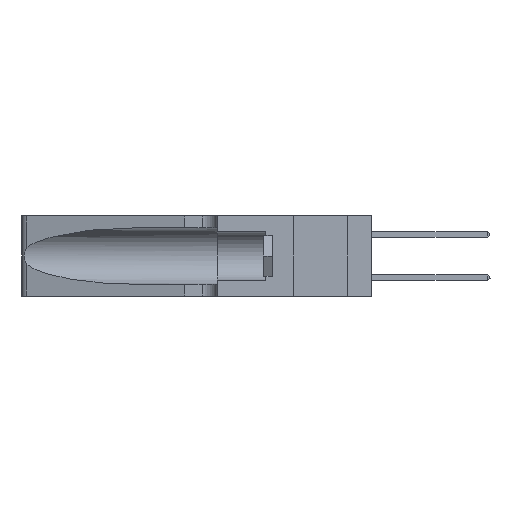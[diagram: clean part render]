
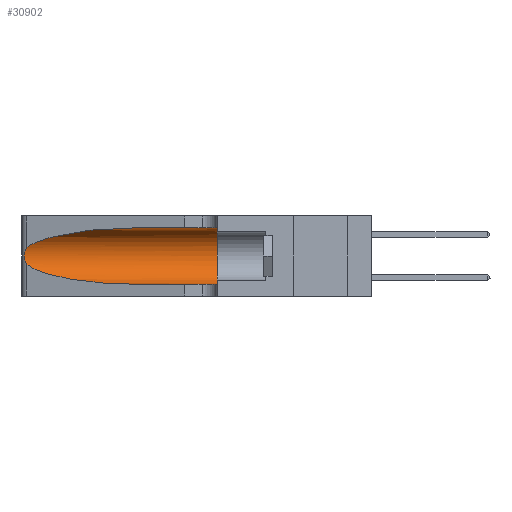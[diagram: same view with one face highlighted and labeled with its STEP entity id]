
A CAD part, left-side view. The second image highlights one B-rep face of the part: STEP entity #30902.
In plain terms, the highlighted cylindrical face has radius 3.308 mm (diameter 6.617 mm), a partial arc.
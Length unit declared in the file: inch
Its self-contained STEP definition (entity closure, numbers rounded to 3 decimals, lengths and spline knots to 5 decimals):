
#442 = AXIS2_PLACEMENT_3D ( 'NONE', #27284, #17613, #19500 ) ;
#1163 = VERTEX_POINT ( 'NONE', #16244 ) ;
#1257 = CARTESIAN_POINT ( 'NONE',  ( 0.25639, 1.23184, 0.21858 ) ) ;
#1404 = CARTESIAN_POINT ( 'NONE',  ( 0.18966, 0.96281, 0.31525 ) ) ;
#1647 = CARTESIAN_POINT ( 'NONE',  ( 0.1305, 0.35, 0.05475 ) ) ;
#2185 = DIRECTION ( 'NONE',  ( 0., -1., 0. ) ) ;
#2292 = ORIENTED_EDGE ( 'NONE', *, *, #30239, .F. ) ;
#2803 = CARTESIAN_POINT ( 'NONE',  ( 0.26018, 1.23835, 0.19895 ) ) ;
#2927 = CARTESIAN_POINT ( 'NONE',  ( 0.25487, 1.22718, 0.22369 ) ) ;
#2942 = B_SPLINE_CURVE_WITH_KNOTS ( 'NONE', 3,
 ( #3809, #17002, #1257, #11878, #21804, #2803, #13673, #11455, #18911, #19011, #21663, #30818, #4128, #14915 ),
 .UNSPECIFIED., .F., .F.,
 ( 4, 2, 2, 2, 2, 2, 4 ),
 ( 0., 0.00027, 0.00053, 0.00107, 0.0016, 0.00187, 0.00214 ),
 .UNSPECIFIED. ) ;
#3809 = CARTESIAN_POINT ( 'NONE',  ( 0.25487, 1.22718, 0.22369 ) ) ;
#4065 = CARTESIAN_POINT ( 'NONE',  ( 0.1305, 0.35, 0.31525 ) ) ;
#4128 = CARTESIAN_POINT ( 'NONE',  ( 0.25555, 1.22993, 0.14849 ) ) ;
#4614 = VECTOR ( 'NONE', #16559, 39.37008 ) ;
#6263 = VERTEX_POINT ( 'NONE', #28391 ) ;
#6730 = DIRECTION ( 'NONE',  ( 0., -1., 0. ) ) ;
#6865 = DIRECTION ( 'NONE',  ( 0., 0., -1. ) ) ;
#7056 = VERTEX_POINT ( 'NONE', #18140 ) ;
#7156 = ORIENTED_EDGE ( 'NONE', *, *, #26812, .T. ) ;
#7515 = CARTESIAN_POINT ( 'NONE',  ( 0.1305, 1.61858, 0.31525 ) ) ;
#7956 = VERTEX_POINT ( 'NONE', #4065 ) ;
#8506 = LINE ( 'NONE', #7515, #19098 ) ;
#10149 =( BOUNDED_CURVE ( )  B_SPLINE_CURVE ( 3, ( #13030, #28681, #33867, #18249 ),
 .UNSPECIFIED., .F., .F. ) 
 B_SPLINE_CURVE_WITH_KNOTS ( ( 4, 4 ),
 ( 3.44316, 4.71239 ),
 .UNSPECIFIED. ) 
 CURVE ( )  GEOMETRIC_REPRESENTATION_ITEM ( )  RATIONAL_B_SPLINE_CURVE ( ( 1., 0.87, 0.87, 1. ) ) 
 REPRESENTATION_ITEM ( '' )  );
#11455 = CARTESIAN_POINT ( 'NONE',  ( 0.26075, 1.23896, 0.178 ) ) ;
#11756 = CARTESIAN_POINT ( 'NONE',  ( 0.2373, 1.15595, 0.28018 ) ) ;
#11878 = CARTESIAN_POINT ( 'NONE',  ( 0.25787, 1.23484, 0.2124 ) ) ;
#13030 = CARTESIAN_POINT ( 'NONE',  ( 0.25487, 1.22718, 0.14631 ) ) ;
#13514 = EDGE_CURVE ( 'NONE', #6263, #29151, #22224, .T. ) ;
#13673 = CARTESIAN_POINT ( 'NONE',  ( 0.26075, 1.23896, 0.19203 ) ) ;
#14915 = CARTESIAN_POINT ( 'NONE',  ( 0.25487, 1.22718, 0.14631 ) ) ;
#15560 = AXIS2_PLACEMENT_3D ( 'NONE', #17385, #6730, #6865 ) ;
#16124 = CARTESIAN_POINT ( 'NONE',  ( 0.1305, 0.72297, 0.31525 ) ) ;
#16244 = CARTESIAN_POINT ( 'NONE',  ( 0.25487, 1.22718, 0.14631 ) ) ;
#16559 = DIRECTION ( 'NONE',  ( 0., -1., 0. ) ) ;
#16983 = VERTEX_POINT ( 'NONE', #1647 ) ;
#17002 = CARTESIAN_POINT ( 'NONE',  ( 0.25555, 1.22994, 0.2215 ) ) ;
#17385 = CARTESIAN_POINT ( 'NONE',  ( 0.1305, 1.61858, 0.185 ) ) ;
#17613 = DIRECTION ( 'NONE',  ( 0., 1., 0. ) ) ;
#18140 = CARTESIAN_POINT ( 'NONE',  ( 0.1305, 0.72297, 0.05475 ) ) ;
#18249 = CARTESIAN_POINT ( 'NONE',  ( 0.1305, 0.72297, 0.05475 ) ) ;
#18911 = CARTESIAN_POINT ( 'NONE',  ( 0.26017, 1.23833, 0.17102 ) ) ;
#19011 = CARTESIAN_POINT ( 'NONE',  ( 0.25856, 1.23593, 0.16098 ) ) ;
#19098 = VECTOR ( 'NONE', #2185, 39.37008 ) ;
#19500 = DIRECTION ( 'NONE',  ( 0., 0., 1. ) ) ;
#20581 = LINE ( 'NONE', #27011, #4614 ) ;
#21357 = EDGE_LOOP ( 'NONE', ( #32444, #26172, #7156, #22757, #29690, #2292 ) ) ;
#21663 = CARTESIAN_POINT ( 'NONE',  ( 0.25789, 1.23486, 0.15765 ) ) ;
#21782 = EDGE_CURVE ( 'NONE', #29151, #1163, #2942, .T. ) ;
#21804 = CARTESIAN_POINT ( 'NONE',  ( 0.25854, 1.2359, 0.20912 ) ) ;
#22224 =( BOUNDED_CURVE ( )  B_SPLINE_CURVE ( 3, ( #16124, #1404, #11756, #30199 ),
 .UNSPECIFIED., .F., .T. ) 
 B_SPLINE_CURVE_WITH_KNOTS ( ( 4, 4 ),
 ( 1.5708, 2.84003 ),
 .UNSPECIFIED. ) 
 CURVE ( )  GEOMETRIC_REPRESENTATION_ITEM ( )  RATIONAL_B_SPLINE_CURVE ( ( 1., 0.87, 0.87, 1. ) ) 
 REPRESENTATION_ITEM ( '' )  );
#22741 = EDGE_CURVE ( 'NONE', #7956, #16983, #33858, .T. ) ;
#22757 = ORIENTED_EDGE ( 'NONE', *, *, #24244, .T. ) ;
#23260 = CYLINDRICAL_SURFACE ( 'NONE', #15560, 0.13025 ) ;
#24244 = EDGE_CURVE ( 'NONE', #7056, #16983, #20581, .T. ) ;
#26172 = ORIENTED_EDGE ( 'NONE', *, *, #21782, .T. ) ;
#26812 = EDGE_CURVE ( 'NONE', #1163, #7056, #10149, .T. ) ;
#27011 = CARTESIAN_POINT ( 'NONE',  ( 0.1305, 1.61858, 0.05475 ) ) ;
#27284 = CARTESIAN_POINT ( 'NONE',  ( 0.1305, 0.35, 0.185 ) ) ;
#27701 = FACE_OUTER_BOUND ( 'NONE', #21357, .T. ) ;
#28391 = CARTESIAN_POINT ( 'NONE',  ( 0.1305, 0.72297, 0.31525 ) ) ;
#28681 = CARTESIAN_POINT ( 'NONE',  ( 0.2373, 1.15595, 0.08982 ) ) ;
#29151 = VERTEX_POINT ( 'NONE', #2927 ) ;
#29690 = ORIENTED_EDGE ( 'NONE', *, *, #22741, .F. ) ;
#30199 = CARTESIAN_POINT ( 'NONE',  ( 0.25487, 1.22718, 0.22369 ) ) ;
#30239 = EDGE_CURVE ( 'NONE', #6263, #7956, #8506, .T. ) ;
#30818 = CARTESIAN_POINT ( 'NONE',  ( 0.25639, 1.23186, 0.15144 ) ) ;
#30902 = ADVANCED_FACE ( 'NONE', ( #27701 ), #23260, .F. ) ;
#32444 = ORIENTED_EDGE ( 'NONE', *, *, #13514, .T. ) ;
#33858 = CIRCLE ( 'NONE', #442, 0.13025 ) ;
#33867 = CARTESIAN_POINT ( 'NONE',  ( 0.18966, 0.96281, 0.05475 ) ) ;
